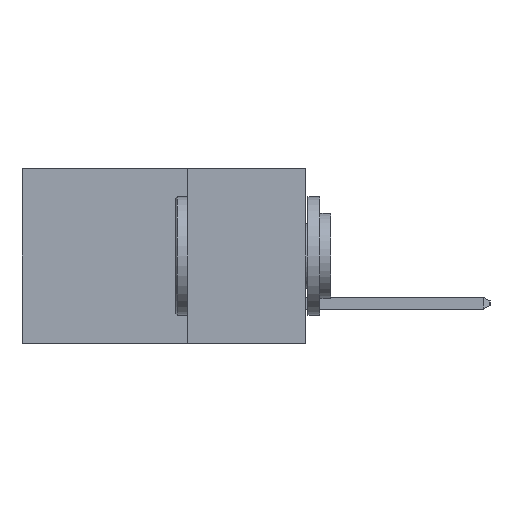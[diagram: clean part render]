
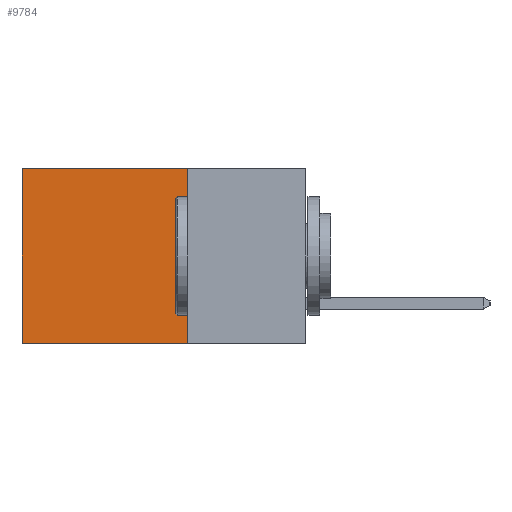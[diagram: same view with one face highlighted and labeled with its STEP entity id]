
A CAD part, left-side view. The second image highlights one B-rep face of the part: STEP entity #9784.
In plain terms, the highlighted planar face has unit normal (-1, 0, 0).
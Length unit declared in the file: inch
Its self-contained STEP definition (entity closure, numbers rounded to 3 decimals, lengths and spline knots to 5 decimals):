
#296 = ORIENTED_EDGE ( 'NONE', *, *, #7024, .T. ) ;
#479 = DIRECTION ( 'NONE',  ( 0., 1., 0. ) ) ;
#1488 = DIRECTION ( 'NONE',  ( 0., 0., -1. ) ) ;
#2539 = PLANE ( 'NONE',  #12991 ) ;
#2621 = ORIENTED_EDGE ( 'NONE', *, *, #14683, .F. ) ;
#2723 = DIRECTION ( 'NONE',  ( 0., 1., 0. ) ) ;
#2851 = CARTESIAN_POINT ( 'NONE',  ( 0.298, 0.25, 0. ) ) ;
#3163 = LINE ( 'NONE', #2851, #8980 ) ;
#3631 = CARTESIAN_POINT ( 'NONE',  ( 0.298, 0.6, -0.37 ) ) ;
#3969 = LINE ( 'NONE', #13410, #12734 ) ;
#4912 = DIRECTION ( 'NONE',  ( 1., 0., 0. ) ) ;
#5049 = CARTESIAN_POINT ( 'NONE',  ( 0.298, 0.25, 0. ) ) ;
#5118 = CARTESIAN_POINT ( 'NONE',  ( 0.298, 0.25, -0.37 ) ) ;
#5360 = VECTOR ( 'NONE', #479, 39.37008 ) ;
#5365 = EDGE_CURVE ( 'NONE', #6736, #11465, #3163, .T. ) ;
#6464 = EDGE_LOOP ( 'NONE', ( #296, #13871, #2621, #9049 ) ) ;
#6736 = VERTEX_POINT ( 'NONE', #5049 ) ;
#7024 = EDGE_CURVE ( 'NONE', #11465, #9736, #3969, .T. ) ;
#8416 = LINE ( 'NONE', #5118, #5360 ) ;
#8450 = FACE_OUTER_BOUND ( 'NONE', #6464, .T. ) ;
#8797 = CARTESIAN_POINT ( 'NONE',  ( 0.298, 0.25, -0.37 ) ) ;
#8812 = VERTEX_POINT ( 'NONE', #8797 ) ;
#8980 = VECTOR ( 'NONE', #2723, 39.37008 ) ;
#9049 = ORIENTED_EDGE ( 'NONE', *, *, #5365, .T. ) ;
#9606 = VECTOR ( 'NONE', #1488, 39.37008 ) ;
#9736 = VERTEX_POINT ( 'NONE', #3631 ) ;
#9784 = ADVANCED_FACE ( 'NONE', ( #8450 ), #2539, .F. ) ;
#9976 = LINE ( 'NONE', #12958, #9606 ) ;
#10612 = EDGE_CURVE ( 'NONE', #8812, #9736, #8416, .T. ) ;
#11465 = VERTEX_POINT ( 'NONE', #12010 ) ;
#11769 = CARTESIAN_POINT ( 'NONE',  ( 0.298, 0.25, 0. ) ) ;
#12010 = CARTESIAN_POINT ( 'NONE',  ( 0.298, 0.6, 0. ) ) ;
#12326 = DIRECTION ( 'NONE',  ( 0., 0., -1. ) ) ;
#12734 = VECTOR ( 'NONE', #12326, 39.37008 ) ;
#12888 = DIRECTION ( 'NONE',  ( 0., 0., -1. ) ) ;
#12958 = CARTESIAN_POINT ( 'NONE',  ( 0.298, 0.25, 0. ) ) ;
#12991 = AXIS2_PLACEMENT_3D ( 'NONE', #11769, #4912, #12888 ) ;
#13410 = CARTESIAN_POINT ( 'NONE',  ( 0.298, 0.6, 0. ) ) ;
#13871 = ORIENTED_EDGE ( 'NONE', *, *, #10612, .F. ) ;
#14683 = EDGE_CURVE ( 'NONE', #6736, #8812, #9976, .T. ) ;
